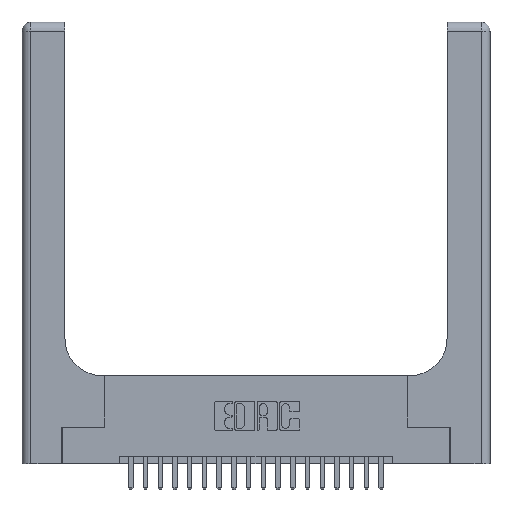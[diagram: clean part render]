
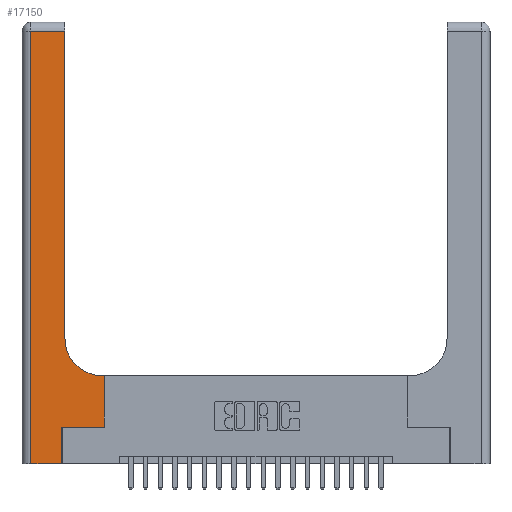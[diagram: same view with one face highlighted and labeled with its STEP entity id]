
A CAD part, top view. The second image highlights one B-rep face of the part: STEP entity #17150.
In plain terms, the highlighted planar face has unit normal (0, 0, 1).
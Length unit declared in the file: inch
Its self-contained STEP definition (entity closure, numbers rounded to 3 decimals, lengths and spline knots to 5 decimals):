
#379 = VECTOR ( 'NONE', #21994, 39.37008 ) ;
#483 = DIRECTION ( 'NONE',  ( 0., 0., -1. ) ) ;
#530 = DIRECTION ( 'NONE',  ( -1., 0., 0. ) ) ;
#636 = CARTESIAN_POINT ( 'NONE',  ( 0.2915, 0.6, 0.37 ) ) ;
#715 = CARTESIAN_POINT ( 'NONE',  ( 0.5415, 0.6, 0.37 ) ) ;
#1297 = CARTESIAN_POINT ( 'NONE',  ( 0.06, 0., 0.37 ) ) ;
#2105 = CARTESIAN_POINT ( 'NONE',  ( 0., 3., 0.37 ) ) ;
#2530 = CARTESIAN_POINT ( 'NONE',  ( 0., 2.94, 0.37 ) ) ;
#2609 = ORIENTED_EDGE ( 'NONE', *, *, #9621, .T. ) ;
#2794 = ORIENTED_EDGE ( 'NONE', *, *, #20464, .T. ) ;
#3151 = CARTESIAN_POINT ( 'NONE',  ( 0.5585, 0.6, 0.37 ) ) ;
#3368 = VERTEX_POINT ( 'NONE', #1297 ) ;
#3398 = EDGE_LOOP ( 'NONE', ( #11039, #16774, #2794, #11050, #10278, #16627, #19726, #20126, #2609 ) ) ;
#3956 = VECTOR ( 'NONE', #22289, 39.37008 ) ;
#4838 = DIRECTION ( 'NONE',  ( 0., 1., 0. ) ) ;
#5048 = LINE ( 'NONE', #7941, #379 ) ;
#5216 = LINE ( 'NONE', #636, #11838 ) ;
#5339 = VERTEX_POINT ( 'NONE', #10295 ) ;
#5887 = EDGE_CURVE ( 'NONE', #17372, #8767, #11262, .T. ) ;
#6241 = DIRECTION ( 'NONE',  ( 0., 1., 0. ) ) ;
#6598 = VECTOR ( 'NONE', #10098, 39.37008 ) ;
#6968 = DIRECTION ( 'NONE',  ( 1., 0., 0. ) ) ;
#7194 = VERTEX_POINT ( 'NONE', #715 ) ;
#7320 = CARTESIAN_POINT ( 'NONE',  ( 0.2915, 0.85, 0.37 ) ) ;
#7587 = EDGE_CURVE ( 'NONE', #17245, #17372, #19318, .T. ) ;
#7941 = CARTESIAN_POINT ( 'NONE',  ( 0.06, 3., 0.37 ) ) ;
#8228 = EDGE_CURVE ( 'NONE', #5339, #17245, #17385, .T. ) ;
#8620 = CARTESIAN_POINT ( 'NONE',  ( 0.269, 0.25, 0.37 ) ) ;
#8767 = VERTEX_POINT ( 'NONE', #3151 ) ;
#9176 = VERTEX_POINT ( 'NONE', #19958 ) ;
#9205 = CARTESIAN_POINT ( 'NONE',  ( 0.5585, 0.25, 0.37 ) ) ;
#9237 = FACE_OUTER_BOUND ( 'NONE', #3398, .T. ) ;
#9621 = EDGE_CURVE ( 'NONE', #7194, #10340, #21692, .T. ) ;
#10098 = DIRECTION ( 'NONE',  ( 0., 1., 0. ) ) ;
#10118 = CARTESIAN_POINT ( 'NONE',  ( 0., 0., 0.37 ) ) ;
#10278 = ORIENTED_EDGE ( 'NONE', *, *, #8228, .T. ) ;
#10295 = CARTESIAN_POINT ( 'NONE',  ( 0.269, 0., 0.37 ) ) ;
#10340 = VERTEX_POINT ( 'NONE', #7320 ) ;
#10618 = VECTOR ( 'NONE', #530, 39.37008 ) ;
#11039 = ORIENTED_EDGE ( 'NONE', *, *, #16099, .T. ) ;
#11050 = ORIENTED_EDGE ( 'NONE', *, *, #20620, .T. ) ;
#11262 = LINE ( 'NONE', #16802, #6598 ) ;
#11718 = EDGE_CURVE ( 'NONE', #8767, #7194, #5216, .T. ) ;
#11838 = VECTOR ( 'NONE', #12936, 39.37008 ) ;
#11969 = VECTOR ( 'NONE', #4838, 39.37008 ) ;
#12427 = CARTESIAN_POINT ( 'NONE',  ( 0.5415, 0.85, 0.37 ) ) ;
#12936 = DIRECTION ( 'NONE',  ( -1., 0., 0. ) ) ;
#12938 = DIRECTION ( 'NONE',  ( -1., 0., 0. ) ) ;
#13141 = CARTESIAN_POINT ( 'NONE',  ( 0.2915, 3., 0.37 ) ) ;
#13444 = VERTEX_POINT ( 'NONE', #13779 ) ;
#13779 = CARTESIAN_POINT ( 'NONE',  ( 0.2915, 2.94, 0.37 ) ) ;
#14443 = CARTESIAN_POINT ( 'NONE',  ( 0.269, 0.25, 0.37 ) ) ;
#14711 = VECTOR ( 'NONE', #19127, 39.37008 ) ;
#15290 = VECTOR ( 'NONE', #6241, 39.37008 ) ;
#15445 = LINE ( 'NONE', #10118, #3956 ) ;
#15872 = AXIS2_PLACEMENT_3D ( 'NONE', #12427, #21187, #6968 ) ;
#16099 = EDGE_CURVE ( 'NONE', #10340, #13444, #19079, .T. ) ;
#16627 = ORIENTED_EDGE ( 'NONE', *, *, #7587, .T. ) ;
#16774 = ORIENTED_EDGE ( 'NONE', *, *, #18592, .T. ) ;
#16802 = CARTESIAN_POINT ( 'NONE',  ( 0.5585, 0.25, 0.37 ) ) ;
#17150 = ADVANCED_FACE ( 'NONE', ( #9237 ), #19838, .F. ) ;
#17245 = VERTEX_POINT ( 'NONE', #14443 ) ;
#17356 = CARTESIAN_POINT ( 'NONE',  ( 0.269, 0., 0.37 ) ) ;
#17372 = VERTEX_POINT ( 'NONE', #9205 ) ;
#17385 = LINE ( 'NONE', #17356, #11969 ) ;
#18592 = EDGE_CURVE ( 'NONE', #13444, #9176, #20411, .T. ) ;
#19079 = LINE ( 'NONE', #13141, #15290 ) ;
#19127 = DIRECTION ( 'NONE',  ( 1., 0., 0. ) ) ;
#19318 = LINE ( 'NONE', #8620, #14711 ) ;
#19726 = ORIENTED_EDGE ( 'NONE', *, *, #5887, .T. ) ;
#19838 = PLANE ( 'NONE',  #22220 ) ;
#19958 = CARTESIAN_POINT ( 'NONE',  ( 0.06, 2.94, 0.37 ) ) ;
#20126 = ORIENTED_EDGE ( 'NONE', *, *, #11718, .T. ) ;
#20411 = LINE ( 'NONE', #2530, #10618 ) ;
#20464 = EDGE_CURVE ( 'NONE', #9176, #3368, #5048, .T. ) ;
#20620 = EDGE_CURVE ( 'NONE', #3368, #5339, #15445, .T. ) ;
#21187 = DIRECTION ( 'NONE',  ( 0., 0., -1. ) ) ;
#21692 = CIRCLE ( 'NONE', #15872, 0.25 ) ;
#21994 = DIRECTION ( 'NONE',  ( 0., -1., 0. ) ) ;
#22220 = AXIS2_PLACEMENT_3D ( 'NONE', #2105, #483, #12938 ) ;
#22289 = DIRECTION ( 'NONE',  ( 1., 0., 0. ) ) ;
